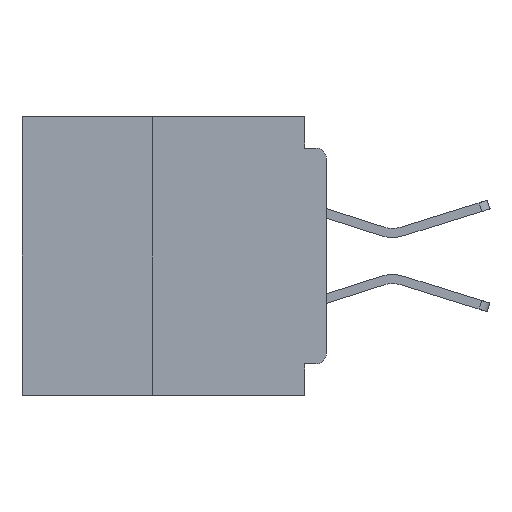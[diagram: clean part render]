
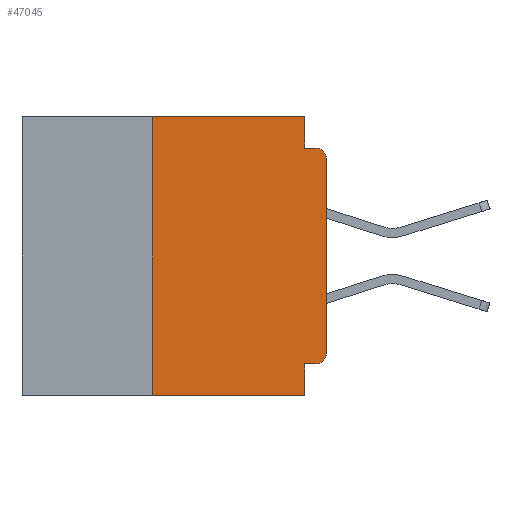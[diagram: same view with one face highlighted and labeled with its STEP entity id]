
A CAD part, left-side view. The second image highlights one B-rep face of the part: STEP entity #47045.
In plain terms, the highlighted planar face has unit normal (-1, 0, 0).
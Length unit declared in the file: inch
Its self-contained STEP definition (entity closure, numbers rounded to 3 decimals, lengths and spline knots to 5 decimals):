
#785 = VECTOR ( 'NONE', #44733, 39.37008 ) ;
#1265 = CARTESIAN_POINT ( 'NONE',  ( 0., 0.437, 0. ) ) ;
#2366 = CARTESIAN_POINT ( 'NONE',  ( 0., 0.015, -0.355 ) ) ;
#2753 = AXIS2_PLACEMENT_3D ( 'NONE', #23329, #50693, #27358 ) ;
#3943 = VECTOR ( 'NONE', #16786, 39.37008 ) ;
#4318 = VECTOR ( 'NONE', #5301, 39.37008 ) ;
#4550 = CARTESIAN_POINT ( 'NONE',  ( 0., 0.015, -0.06 ) ) ;
#5301 = DIRECTION ( 'NONE',  ( 0., -1., 0. ) ) ;
#6529 = ORIENTED_EDGE ( 'NONE', *, *, #46009, .F. ) ;
#7040 = CARTESIAN_POINT ( 'NONE',  ( 0., 0.031, 0. ) ) ;
#7275 = CARTESIAN_POINT ( 'NONE',  ( 0., 0.031, -0.045 ) ) ;
#7478 = DIRECTION ( 'NONE',  ( 1., 0., 0. ) ) ;
#7673 = VERTEX_POINT ( 'NONE', #26044 ) ;
#8557 = DIRECTION ( 'NONE',  ( 0., 0., -1. ) ) ;
#8869 = ORIENTED_EDGE ( 'NONE', *, *, #18385, .T. ) ;
#9339 = VERTEX_POINT ( 'NONE', #24308 ) ;
#9456 = CARTESIAN_POINT ( 'NONE',  ( 0., 0.25, 0. ) ) ;
#10136 = LINE ( 'NONE', #17235, #785 ) ;
#10460 = LINE ( 'NONE', #34491, #19778 ) ;
#11025 = CARTESIAN_POINT ( 'NONE',  ( 0., 0.25, -0.4 ) ) ;
#11194 = VERTEX_POINT ( 'NONE', #13854 ) ;
#11592 = CARTESIAN_POINT ( 'NONE',  ( 0., 0.437, 0. ) ) ;
#12057 = VERTEX_POINT ( 'NONE', #11025 ) ;
#12257 = ORIENTED_EDGE ( 'NONE', *, *, #18308, .F. ) ;
#12378 = DIRECTION ( 'NONE',  ( 0., -1., 0. ) ) ;
#13732 = LINE ( 'NONE', #7040, #42740 ) ;
#13854 = CARTESIAN_POINT ( 'NONE',  ( 0., 0.031, -0.355 ) ) ;
#14277 = CARTESIAN_POINT ( 'NONE',  ( 0., 0.031, 0. ) ) ;
#14348 = VERTEX_POINT ( 'NONE', #9456 ) ;
#14637 = LINE ( 'NONE', #36078, #44789 ) ;
#14758 = DIRECTION ( 'NONE',  ( 0., 0., -1. ) ) ;
#14903 = ORIENTED_EDGE ( 'NONE', *, *, #15570, .F. ) ;
#15570 = EDGE_CURVE ( 'NONE', #19366, #7673, #36746, .T. ) ;
#15577 = PLANE ( 'NONE',  #22852 ) ;
#16605 = EDGE_LOOP ( 'NONE', ( #33838, #30337, #14903, #12257, #6529, #43110, #24429, #22748, #24509, #8869 ) ) ;
#16786 = DIRECTION ( 'NONE',  ( 0., -1., 0. ) ) ;
#17235 = CARTESIAN_POINT ( 'NONE',  ( 0., 0., 0. ) ) ;
#18308 = EDGE_CURVE ( 'NONE', #28329, #19366, #13732, .T. ) ;
#18385 = EDGE_CURVE ( 'NONE', #33890, #9339, #29927, .T. ) ;
#19366 = VERTEX_POINT ( 'NONE', #7275 ) ;
#19593 = DIRECTION ( 'NONE',  ( 0., 0., -1. ) ) ;
#19778 = VECTOR ( 'NONE', #14758, 39.37008 ) ;
#19882 = CARTESIAN_POINT ( 'NONE',  ( 0., 0., -0.06 ) ) ;
#22748 = ORIENTED_EDGE ( 'NONE', *, *, #35188, .F. ) ;
#22852 = AXIS2_PLACEMENT_3D ( 'NONE', #11592, #7478, #19593 ) ;
#23329 = CARTESIAN_POINT ( 'NONE',  ( 0., 0.015, -0.34 ) ) ;
#23909 = AXIS2_PLACEMENT_3D ( 'NONE', #4550, #32269, #8557 ) ;
#24168 = EDGE_CURVE ( 'NONE', #25672, #7673, #43551, .T. ) ;
#24308 = CARTESIAN_POINT ( 'NONE',  ( 0., 0., -0.34 ) ) ;
#24429 = ORIENTED_EDGE ( 'NONE', *, *, #37343, .T. ) ;
#24509 = ORIENTED_EDGE ( 'NONE', *, *, #41770, .F. ) ;
#25672 = VERTEX_POINT ( 'NONE', #19882 ) ;
#26044 = CARTESIAN_POINT ( 'NONE',  ( 0., 0.015, -0.045 ) ) ;
#27358 = DIRECTION ( 'NONE',  ( 0., 0., -1. ) ) ;
#27516 = DIRECTION ( 'NONE',  ( 0., 1., 0. ) ) ;
#28329 = VERTEX_POINT ( 'NONE', #14277 ) ;
#29927 = CIRCLE ( 'NONE', #2753, 0.015 ) ;
#30337 = ORIENTED_EDGE ( 'NONE', *, *, #24168, .T. ) ;
#31484 = LINE ( 'NONE', #35196, #50973 ) ;
#32121 = FACE_OUTER_BOUND ( 'NONE', #16605, .T. ) ;
#32246 = CARTESIAN_POINT ( 'NONE',  ( 0., 0.25, -0.4 ) ) ;
#32269 = DIRECTION ( 'NONE',  ( -1., 0., 0. ) ) ;
#33838 = ORIENTED_EDGE ( 'NONE', *, *, #39578, .T. ) ;
#33890 = VERTEX_POINT ( 'NONE', #2366 ) ;
#34491 = CARTESIAN_POINT ( 'NONE',  ( 0., 0.031, -0.4 ) ) ;
#35188 = EDGE_CURVE ( 'NONE', #11194, #41323, #10460, .T. ) ;
#35196 = CARTESIAN_POINT ( 'NONE',  ( 0., 0., -0.355 ) ) ;
#35905 = LINE ( 'NONE', #1265, #4318 ) ;
#36078 = CARTESIAN_POINT ( 'NONE',  ( 0., 0.437, -0.4 ) ) ;
#36194 = DIRECTION ( 'NONE',  ( 0., 0., 1. ) ) ;
#36746 = LINE ( 'NONE', #48236, #3943 ) ;
#37343 = EDGE_CURVE ( 'NONE', #12057, #41323, #14637, .T. ) ;
#38621 = DIRECTION ( 'NONE',  ( 0., 0., -1. ) ) ;
#39097 = LINE ( 'NONE', #32246, #48252 ) ;
#39578 = EDGE_CURVE ( 'NONE', #9339, #25672, #10136, .T. ) ;
#40157 = EDGE_CURVE ( 'NONE', #12057, #14348, #39097, .T. ) ;
#41323 = VERTEX_POINT ( 'NONE', #43252 ) ;
#41770 = EDGE_CURVE ( 'NONE', #33890, #11194, #31484, .T. ) ;
#42740 = VECTOR ( 'NONE', #38621, 39.37008 ) ;
#43110 = ORIENTED_EDGE ( 'NONE', *, *, #40157, .F. ) ;
#43252 = CARTESIAN_POINT ( 'NONE',  ( 0., 0.031, -0.4 ) ) ;
#43551 = CIRCLE ( 'NONE', #23909, 0.015 ) ;
#44733 = DIRECTION ( 'NONE',  ( 0., 0., 1. ) ) ;
#44789 = VECTOR ( 'NONE', #12378, 39.37008 ) ;
#46009 = EDGE_CURVE ( 'NONE', #14348, #28329, #35905, .T. ) ;
#47045 = ADVANCED_FACE ( 'NONE', ( #32121 ), #15577, .F. ) ;
#48236 = CARTESIAN_POINT ( 'NONE',  ( 0., 0., -0.045 ) ) ;
#48252 = VECTOR ( 'NONE', #36194, 39.37008 ) ;
#50693 = DIRECTION ( 'NONE',  ( -1., 0., 0. ) ) ;
#50973 = VECTOR ( 'NONE', #27516, 39.37008 ) ;
